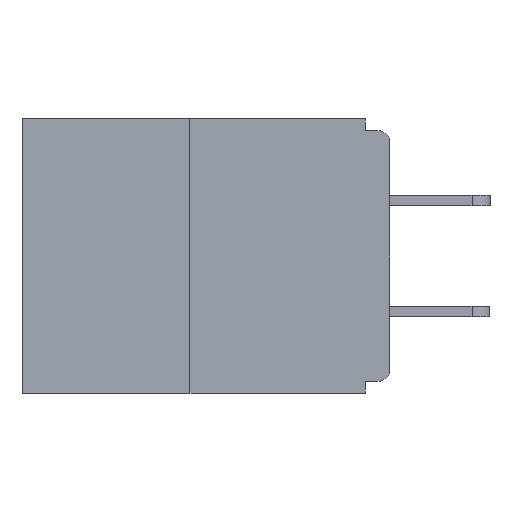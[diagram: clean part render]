
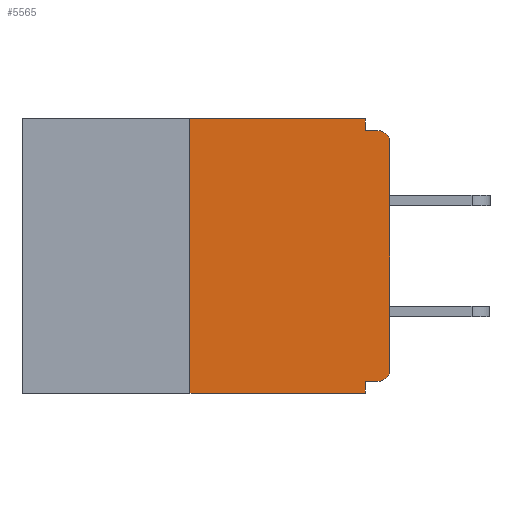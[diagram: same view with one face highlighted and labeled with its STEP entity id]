
A CAD part, left-side view. The second image highlights one B-rep face of the part: STEP entity #5565.
In plain terms, the highlighted planar face has unit normal (-1, 0, 0).
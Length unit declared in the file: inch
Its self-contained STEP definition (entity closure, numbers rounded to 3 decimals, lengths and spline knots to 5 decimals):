
#99 = DIRECTION ( 'NONE',  ( 0., 0., -1. ) ) ;
#153 = LINE ( 'NONE', #5926, #9508 ) ;
#409 = DIRECTION ( 'NONE',  ( 0., 1., 0. ) ) ;
#625 = EDGE_CURVE ( 'NONE', #6089, #1886, #13655, .T. ) ;
#1047 = CARTESIAN_POINT ( 'NONE',  ( 0., 0.015, -0.03 ) ) ;
#1082 = LINE ( 'NONE', #3658, #14875 ) ;
#1093 = VECTOR ( 'NONE', #409, 39.37008 ) ;
#1332 = EDGE_CURVE ( 'NONE', #10376, #15405, #5343, .T. ) ;
#1674 = ORIENTED_EDGE ( 'NONE', *, *, #2381, .F. ) ;
#1837 = CARTESIAN_POINT ( 'NONE',  ( 0., 0., -0.313 ) ) ;
#1886 = VERTEX_POINT ( 'NONE', #15203 ) ;
#2310 = VECTOR ( 'NONE', #15000, 39.37008 ) ;
#2381 = EDGE_CURVE ( 'NONE', #10762, #8910, #13975, .T. ) ;
#2405 = DIRECTION ( 'NONE',  ( 0., 0., -1. ) ) ;
#2529 = CARTESIAN_POINT ( 'NONE',  ( 0., 0.031, -0.343 ) ) ;
#2707 = AXIS2_PLACEMENT_3D ( 'NONE', #1047, #9778, #2405 ) ;
#2727 = CARTESIAN_POINT ( 'NONE',  ( 0., 0., -0.015 ) ) ;
#2759 = EDGE_CURVE ( 'NONE', #11545, #1886, #7410, .T. ) ;
#2796 = ORIENTED_EDGE ( 'NONE', *, *, #11244, .F. ) ;
#2870 = LINE ( 'NONE', #3395, #9817 ) ;
#2998 = ORIENTED_EDGE ( 'NONE', *, *, #10546, .F. ) ;
#3196 = AXIS2_PLACEMENT_3D ( 'NONE', #12191, #8601, #3570 ) ;
#3395 = CARTESIAN_POINT ( 'NONE',  ( 0., 0.031, 0. ) ) ;
#3570 = DIRECTION ( 'NONE',  ( 0., 0., -1. ) ) ;
#3658 = CARTESIAN_POINT ( 'NONE',  ( 0., 0., 0. ) ) ;
#3709 = PLANE ( 'NONE',  #11234 ) ;
#3967 = CARTESIAN_POINT ( 'NONE',  ( 0., 0., -0.328 ) ) ;
#4616 = EDGE_CURVE ( 'NONE', #10376, #6785, #5084, .T. ) ;
#5084 = LINE ( 'NONE', #3967, #1093 ) ;
#5343 = CIRCLE ( 'NONE', #3196, 0.015 ) ;
#5565 = ADVANCED_FACE ( 'NONE', ( #14108 ), #3709, .F. ) ;
#5573 = CARTESIAN_POINT ( 'NONE',  ( 0., 0.031, -0.015 ) ) ;
#5926 = CARTESIAN_POINT ( 'NONE',  ( 0., 0.46, -0.343 ) ) ;
#6089 = VERTEX_POINT ( 'NONE', #5573 ) ;
#6223 = DIRECTION ( 'NONE',  ( 0., 0., 1. ) ) ;
#6253 = VECTOR ( 'NONE', #12748, 39.37008 ) ;
#6363 = LINE ( 'NONE', #9517, #7709 ) ;
#6641 = EDGE_CURVE ( 'NONE', #8910, #6089, #2870, .T. ) ;
#6785 = VERTEX_POINT ( 'NONE', #7405 ) ;
#6986 = CARTESIAN_POINT ( 'NONE',  ( 0., 0.46, 0. ) ) ;
#7219 = ORIENTED_EDGE ( 'NONE', *, *, #4616, .F. ) ;
#7300 = DIRECTION ( 'NONE',  ( 0., 0., -1. ) ) ;
#7405 = CARTESIAN_POINT ( 'NONE',  ( 0., 0.031, -0.328 ) ) ;
#7410 = CIRCLE ( 'NONE', #2707, 0.015 ) ;
#7709 = VECTOR ( 'NONE', #12124, 39.37008 ) ;
#7730 = CARTESIAN_POINT ( 'NONE',  ( 0., 0.015, -0.328 ) ) ;
#7952 = VECTOR ( 'NONE', #15534, 39.37008 ) ;
#7992 = VERTEX_POINT ( 'NONE', #2529 ) ;
#8144 = CARTESIAN_POINT ( 'NONE',  ( 0., 0.031, -0.343 ) ) ;
#8601 = DIRECTION ( 'NONE',  ( -1., 0., 0. ) ) ;
#8910 = VERTEX_POINT ( 'NONE', #12008 ) ;
#9096 = EDGE_LOOP ( 'NONE', ( #1674, #2796, #10705, #2998, #7219, #10867, #12707, #9130, #11997, #14102 ) ) ;
#9130 = ORIENTED_EDGE ( 'NONE', *, *, #2759, .T. ) ;
#9169 = CARTESIAN_POINT ( 'NONE',  ( 0., 0.25, -0.343 ) ) ;
#9508 = VECTOR ( 'NONE', #15754, 39.37008 ) ;
#9517 = CARTESIAN_POINT ( 'NONE',  ( 0., 0.25, 0. ) ) ;
#9526 = LINE ( 'NONE', #8144, #7952 ) ;
#9778 = DIRECTION ( 'NONE',  ( -1., 0., 0. ) ) ;
#9817 = VECTOR ( 'NONE', #99, 39.37008 ) ;
#10277 = EDGE_CURVE ( 'NONE', #15405, #11545, #1082, .T. ) ;
#10376 = VERTEX_POINT ( 'NONE', #7730 ) ;
#10546 = EDGE_CURVE ( 'NONE', #6785, #7992, #9526, .T. ) ;
#10705 = ORIENTED_EDGE ( 'NONE', *, *, #10875, .T. ) ;
#10762 = VERTEX_POINT ( 'NONE', #13885 ) ;
#10807 = VERTEX_POINT ( 'NONE', #9169 ) ;
#10847 = CARTESIAN_POINT ( 'NONE',  ( 0., 0., -0.03 ) ) ;
#10867 = ORIENTED_EDGE ( 'NONE', *, *, #1332, .T. ) ;
#10875 = EDGE_CURVE ( 'NONE', #10807, #7992, #153, .T. ) ;
#11234 = AXIS2_PLACEMENT_3D ( 'NONE', #13440, #12433, #7300 ) ;
#11244 = EDGE_CURVE ( 'NONE', #10807, #10762, #6363, .T. ) ;
#11545 = VERTEX_POINT ( 'NONE', #10847 ) ;
#11997 = ORIENTED_EDGE ( 'NONE', *, *, #625, .F. ) ;
#12008 = CARTESIAN_POINT ( 'NONE',  ( 0., 0.031, 0. ) ) ;
#12124 = DIRECTION ( 'NONE',  ( 0., 0., 1. ) ) ;
#12191 = CARTESIAN_POINT ( 'NONE',  ( 0., 0.015, -0.313 ) ) ;
#12433 = DIRECTION ( 'NONE',  ( 1., 0., 0. ) ) ;
#12707 = ORIENTED_EDGE ( 'NONE', *, *, #10277, .T. ) ;
#12748 = DIRECTION ( 'NONE',  ( 0., -1., 0. ) ) ;
#13440 = CARTESIAN_POINT ( 'NONE',  ( 0., 0.46, 0. ) ) ;
#13655 = LINE ( 'NONE', #2727, #2310 ) ;
#13885 = CARTESIAN_POINT ( 'NONE',  ( 0., 0.25, 0. ) ) ;
#13975 = LINE ( 'NONE', #6986, #6253 ) ;
#14102 = ORIENTED_EDGE ( 'NONE', *, *, #6641, .F. ) ;
#14108 = FACE_OUTER_BOUND ( 'NONE', #9096, .T. ) ;
#14875 = VECTOR ( 'NONE', #6223, 39.37008 ) ;
#15000 = DIRECTION ( 'NONE',  ( 0., -1., 0. ) ) ;
#15203 = CARTESIAN_POINT ( 'NONE',  ( 0., 0.015, -0.015 ) ) ;
#15405 = VERTEX_POINT ( 'NONE', #1837 ) ;
#15534 = DIRECTION ( 'NONE',  ( 0., 0., -1. ) ) ;
#15754 = DIRECTION ( 'NONE',  ( 0., -1., 0. ) ) ;
